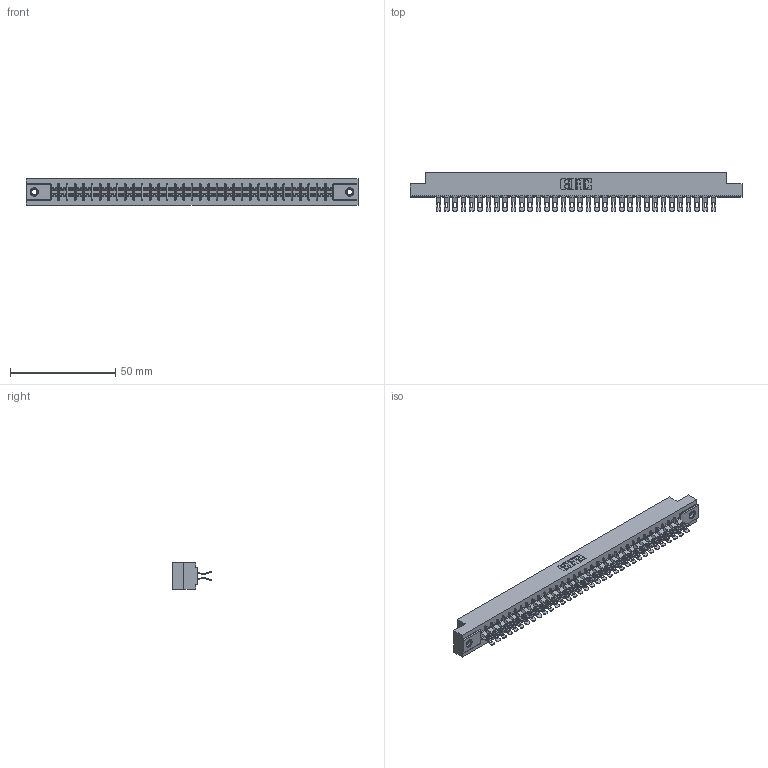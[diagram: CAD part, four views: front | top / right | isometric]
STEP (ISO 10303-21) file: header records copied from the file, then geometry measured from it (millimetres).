
FILE_DESCRIPTION (( 'STEP AP203' ), '1' );
FILE_NAME ('305-068-555-507.STEP', '2019-09-10T04:39:19', ( '' ), ( '' ), 'SwSTEP 2.0', 'SolidWorks 2016', '' );
FILE_SCHEMA (( 'CONFIG_CONTROL_DESIGN' ));
Length unit declared in the file: inch
Products named in the file (4): 345-250-001_345-250-005-103; 305-068-555-507; 305 Part_.156 Dia; 305-290-001_555
Assembly tree (71 placements, depth 2):
  305-068-555-507
    305 Part_.156 Dia
    305-290-001_555  x68
    345-250-001_345-250-005-103  x2
Bounding box: 157.73 x 18.41 x 12.7 mm (x, y, z)
Volume: 16124.2 mm3; surface area: 22398.8 mm2
Topology: 71 solids, 71 shells, 4664 faces, 13882 edges, 9064 vertices
Faces by surface type: plane 2276, cylinder 2236, sphere 136, cone 12, torus 4
Entity records: 39596 total; most frequent: CARTESIAN_POINT 6553, ORIENTED_EDGE 6488, DIRECTION 6350, EDGE_CURVE 3244, VECTOR 2592, LINE 2592, VERTEX_POINT 2066, AXIS2_PLACEMENT_3D 1879
